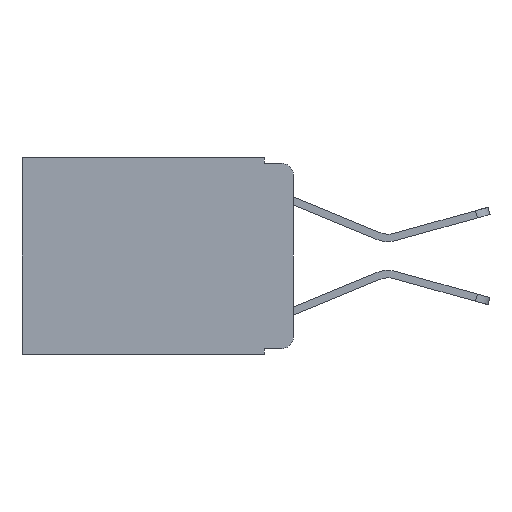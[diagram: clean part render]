
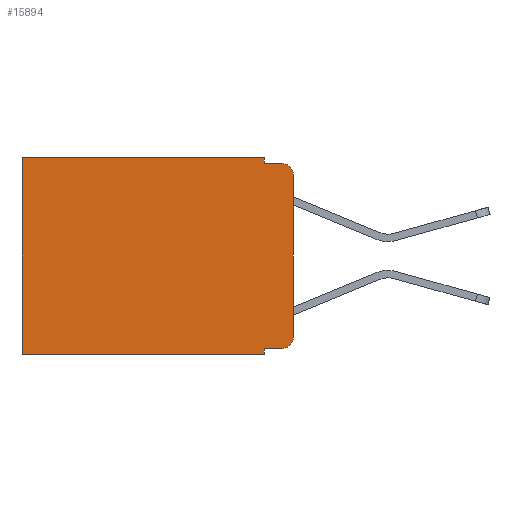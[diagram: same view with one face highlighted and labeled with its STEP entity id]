
A CAD part, left-side view. The second image highlights one B-rep face of the part: STEP entity #15894.
In plain terms, the highlighted planar face has unit normal (-1, 0, 0).
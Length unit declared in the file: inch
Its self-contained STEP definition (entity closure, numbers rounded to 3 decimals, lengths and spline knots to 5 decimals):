
#291 = CARTESIAN_POINT ( 'NONE',  ( 0.298, 0.02, -0.313 ) ) ;
#1012 = CARTESIAN_POINT ( 'NONE',  ( 0.298, 0.051, 0. ) ) ;
#1436 = EDGE_CURVE ( 'NONE', #1908, #14122, #18386, .T. ) ;
#1501 = DIRECTION ( 'NONE',  ( 0., 1., 0. ) ) ;
#1575 = CARTESIAN_POINT ( 'NONE',  ( 0.298, 0., 0. ) ) ;
#1807 = DIRECTION ( 'NONE',  ( 0., 0., -1. ) ) ;
#1908 = VERTEX_POINT ( 'NONE', #9904 ) ;
#2639 = DIRECTION ( 'NONE',  ( 0., -1., 0. ) ) ;
#2643 = VERTEX_POINT ( 'NONE', #7459 ) ;
#2739 = VECTOR ( 'NONE', #5885, 39.37008 ) ;
#2745 = ORIENTED_EDGE ( 'NONE', *, *, #8362, .F. ) ;
#2760 = VECTOR ( 'NONE', #4874, 39.37008 ) ;
#2961 = DIRECTION ( 'NONE',  ( -1., 0., 0. ) ) ;
#3109 = DIRECTION ( 'NONE',  ( 0., 0., -1. ) ) ;
#3112 = ORIENTED_EDGE ( 'NONE', *, *, #14458, .T. ) ;
#3170 = CARTESIAN_POINT ( 'NONE',  ( 0.298, 0.02, -0.333 ) ) ;
#3307 = LINE ( 'NONE', #4160, #14408 ) ;
#3602 = VERTEX_POINT ( 'NONE', #9476 ) ;
#4011 = VERTEX_POINT ( 'NONE', #4612 ) ;
#4160 = CARTESIAN_POINT ( 'NONE',  ( 0.298, 0.051, -0.01 ) ) ;
#4612 = CARTESIAN_POINT ( 'NONE',  ( 0.298, 0.051, -0.333 ) ) ;
#4802 = CARTESIAN_POINT ( 'NONE',  ( 0.298, 0., 0. ) ) ;
#4874 = DIRECTION ( 'NONE',  ( 0., 1., 0. ) ) ;
#5195 = DIRECTION ( 'NONE',  ( 1., 0., 0. ) ) ;
#5222 = CIRCLE ( 'NONE', #14186, 0.02 ) ;
#5885 = DIRECTION ( 'NONE',  ( 0., 0., -1. ) ) ;
#6437 = EDGE_CURVE ( 'NONE', #4011, #15698, #12980, .T. ) ;
#6483 = ORIENTED_EDGE ( 'NONE', *, *, #12282, .T. ) ;
#7027 = DIRECTION ( 'NONE',  ( 0., 0., -1. ) ) ;
#7459 = CARTESIAN_POINT ( 'NONE',  ( 0.298, 0.051, -0.01 ) ) ;
#7703 = ORIENTED_EDGE ( 'NONE', *, *, #10980, .F. ) ;
#8158 = CARTESIAN_POINT ( 'NONE',  ( 0.298, 0.473, -0.343 ) ) ;
#8362 = EDGE_CURVE ( 'NONE', #17237, #2643, #18685, .T. ) ;
#9388 = CARTESIAN_POINT ( 'NONE',  ( 0.298, 0.473, 0. ) ) ;
#9476 = CARTESIAN_POINT ( 'NONE',  ( 0.298, 0.02, -0.01 ) ) ;
#9904 = CARTESIAN_POINT ( 'NONE',  ( 0.298, 0., -0.03 ) ) ;
#9944 = AXIS2_PLACEMENT_3D ( 'NONE', #11651, #2961, #13106 ) ;
#10292 = CARTESIAN_POINT ( 'NONE',  ( 0.298, 0., -0.343 ) ) ;
#10518 = LINE ( 'NONE', #4802, #2760 ) ;
#10520 = EDGE_CURVE ( 'NONE', #17237, #12513, #10518, .T. ) ;
#10581 = DIRECTION ( 'NONE',  ( -1., 0., 0. ) ) ;
#10905 = PLANE ( 'NONE',  #15277 ) ;
#10980 = EDGE_CURVE ( 'NONE', #4011, #17688, #18090, .T. ) ;
#11251 = EDGE_CURVE ( 'NONE', #12513, #14018, #16537, .T. ) ;
#11381 = DIRECTION ( 'NONE',  ( 0., -1., 0. ) ) ;
#11651 = CARTESIAN_POINT ( 'NONE',  ( 0.298, 0.02, -0.03 ) ) ;
#11963 = ORIENTED_EDGE ( 'NONE', *, *, #6437, .T. ) ;
#12282 = EDGE_CURVE ( 'NONE', #1908, #3602, #15184, .T. ) ;
#12513 = VERTEX_POINT ( 'NONE', #16658 ) ;
#12734 = VECTOR ( 'NONE', #17937, 39.37008 ) ;
#12980 = LINE ( 'NONE', #18484, #16348 ) ;
#13106 = DIRECTION ( 'NONE',  ( 0., 0., -1. ) ) ;
#13171 = CARTESIAN_POINT ( 'NONE',  ( 0.298, 0.051, -0.343 ) ) ;
#13816 = CARTESIAN_POINT ( 'NONE',  ( 0.298, 0., 0. ) ) ;
#14018 = VERTEX_POINT ( 'NONE', #8158 ) ;
#14122 = VERTEX_POINT ( 'NONE', #18370 ) ;
#14139 = ORIENTED_EDGE ( 'NONE', *, *, #15473, .F. ) ;
#14186 = AXIS2_PLACEMENT_3D ( 'NONE', #291, #10581, #1807 ) ;
#14339 = ORIENTED_EDGE ( 'NONE', *, *, #11251, .T. ) ;
#14408 = VECTOR ( 'NONE', #2639, 39.37008 ) ;
#14458 = EDGE_CURVE ( 'NONE', #15698, #14122, #5222, .T. ) ;
#14551 = ORIENTED_EDGE ( 'NONE', *, *, #1436, .F. ) ;
#14939 = ORIENTED_EDGE ( 'NONE', *, *, #15613, .F. ) ;
#14946 = VECTOR ( 'NONE', #7027, 39.37008 ) ;
#15184 = CIRCLE ( 'NONE', #9944, 0.02 ) ;
#15248 = DIRECTION ( 'NONE',  ( 0., 0., -1. ) ) ;
#15277 = AXIS2_PLACEMENT_3D ( 'NONE', #13816, #5195, #15248 ) ;
#15473 = EDGE_CURVE ( 'NONE', #2643, #3602, #3307, .T. ) ;
#15517 = LINE ( 'NONE', #10292, #16401 ) ;
#15613 = EDGE_CURVE ( 'NONE', #17688, #14018, #15517, .T. ) ;
#15698 = VERTEX_POINT ( 'NONE', #3170 ) ;
#15894 = ADVANCED_FACE ( 'NONE', ( #18144 ), #10905, .F. ) ;
#16348 = VECTOR ( 'NONE', #11381, 39.37008 ) ;
#16352 = EDGE_LOOP ( 'NONE', ( #14551, #6483, #14139, #2745, #17203, #14339, #14939, #7703, #11963, #3112 ) ) ;
#16401 = VECTOR ( 'NONE', #1501, 39.37008 ) ;
#16494 = CARTESIAN_POINT ( 'NONE',  ( 0.298, 0.051, 0. ) ) ;
#16537 = LINE ( 'NONE', #9388, #12734 ) ;
#16658 = CARTESIAN_POINT ( 'NONE',  ( 0.298, 0.473, 0. ) ) ;
#17203 = ORIENTED_EDGE ( 'NONE', *, *, #10520, .T. ) ;
#17237 = VERTEX_POINT ( 'NONE', #16494 ) ;
#17315 = CARTESIAN_POINT ( 'NONE',  ( 0.298, 0.051, 0. ) ) ;
#17688 = VERTEX_POINT ( 'NONE', #13171 ) ;
#17937 = DIRECTION ( 'NONE',  ( 0., 0., -1. ) ) ;
#17966 = VECTOR ( 'NONE', #3109, 39.37008 ) ;
#18090 = LINE ( 'NONE', #17315, #2739 ) ;
#18144 = FACE_OUTER_BOUND ( 'NONE', #16352, .T. ) ;
#18370 = CARTESIAN_POINT ( 'NONE',  ( 0.298, 0., -0.313 ) ) ;
#18386 = LINE ( 'NONE', #1575, #17966 ) ;
#18484 = CARTESIAN_POINT ( 'NONE',  ( 0.298, 0.051, -0.333 ) ) ;
#18685 = LINE ( 'NONE', #1012, #14946 ) ;
